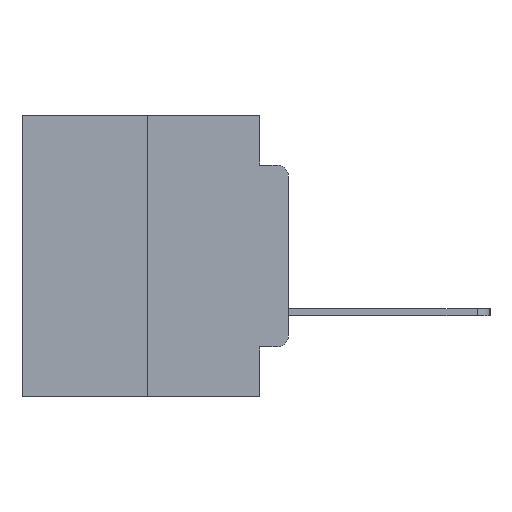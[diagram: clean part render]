
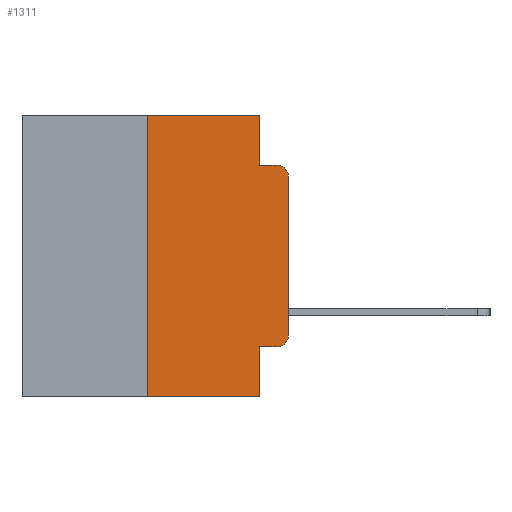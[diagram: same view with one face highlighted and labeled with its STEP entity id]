
A CAD part, left-side view. The second image highlights one B-rep face of the part: STEP entity #1311.
In plain terms, the highlighted planar face has unit normal (-1, 0, 0).
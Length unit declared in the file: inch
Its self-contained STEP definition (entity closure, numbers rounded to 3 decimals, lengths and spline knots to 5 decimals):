
#98 = DIRECTION ( 'NONE',  ( 1., 0., 0. ) ) ;
#114 = DIRECTION ( 'NONE',  ( 0., -1., 0. ) ) ;
#141 = ORIENTED_EDGE ( 'NONE', *, *, #3497, .T. ) ;
#243 = CIRCLE ( 'NONE', #25895, 0.02 ) ;
#265 = ORIENTED_EDGE ( 'NONE', *, *, #6377, .T. ) ;
#320 = ORIENTED_EDGE ( 'NONE', *, *, #17636, .F. ) ;
#381 = FACE_OUTER_BOUND ( 'NONE', #6805, .T. ) ;
#661 = ORIENTED_EDGE ( 'NONE', *, *, #2000, .F. ) ;
#1247 = PLANE ( 'NONE',  #13559 ) ;
#1311 = ADVANCED_FACE ( 'NONE', ( #381 ), #1247, .F. ) ;
#2000 = EDGE_CURVE ( 'NONE', #14058, #24439, #23608, .T. ) ;
#2503 = LINE ( 'NONE', #15978, #13134 ) ;
#2613 = CARTESIAN_POINT ( 'NONE',  ( 0., 0.02, -0.1085 ) ) ;
#2780 = ORIENTED_EDGE ( 'NONE', *, *, #16126, .F. ) ;
#3058 = DIRECTION ( 'NONE',  ( 0., 0., -1. ) ) ;
#3257 = LINE ( 'NONE', #22811, #13185 ) ;
#3497 = EDGE_CURVE ( 'NONE', #26567, #24439, #243, .T. ) ;
#3985 = ORIENTED_EDGE ( 'NONE', *, *, #16803, .T. ) ;
#5022 = ORIENTED_EDGE ( 'NONE', *, *, #11822, .T. ) ;
#5817 = CARTESIAN_POINT ( 'NONE',  ( 0., 0., 0. ) ) ;
#5820 = CIRCLE ( 'NONE', #22094, 0.02 ) ;
#6288 = ORIENTED_EDGE ( 'NONE', *, *, #12007, .F. ) ;
#6369 = VERTEX_POINT ( 'NONE', #16128 ) ;
#6377 = EDGE_CURVE ( 'NONE', #10639, #26567, #12875, .T. ) ;
#6389 = DIRECTION ( 'NONE',  ( -1., 0., 0. ) ) ;
#6685 = CARTESIAN_POINT ( 'NONE',  ( 0., 0.051, -0.0885 ) ) ;
#6805 = EDGE_LOOP ( 'NONE', ( #265, #141, #661, #320, #2780, #17158, #8046, #6288, #5022, #3985 ) ) ;
#8046 = ORIENTED_EDGE ( 'NONE', *, *, #18594, .T. ) ;
#8065 = LINE ( 'NONE', #21687, #18872 ) ;
#8279 = VECTOR ( 'NONE', #17229, 39.37008 ) ;
#8461 = VERTEX_POINT ( 'NONE', #20288 ) ;
#9256 = VECTOR ( 'NONE', #12437, 39.37008 ) ;
#9667 = DIRECTION ( 'NONE',  ( 0., 0., 1. ) ) ;
#10191 = CARTESIAN_POINT ( 'NONE',  ( 0., 0.473, 0. ) ) ;
#10449 = EDGE_CURVE ( 'NONE', #10843, #10741, #8065, .T. ) ;
#10500 = VECTOR ( 'NONE', #26169, 39.37008 ) ;
#10639 = VERTEX_POINT ( 'NONE', #12827 ) ;
#10712 = CARTESIAN_POINT ( 'NONE',  ( 0., 0.02, -0.0885 ) ) ;
#10741 = VERTEX_POINT ( 'NONE', #15293 ) ;
#10785 = CARTESIAN_POINT ( 'NONE',  ( 0., 0.02, -0.3915 ) ) ;
#10843 = VERTEX_POINT ( 'NONE', #21673 ) ;
#10846 = DIRECTION ( 'NONE',  ( 0., 0., -1. ) ) ;
#10914 = VERTEX_POINT ( 'NONE', #23831 ) ;
#11822 = EDGE_CURVE ( 'NONE', #6369, #10914, #25566, .T. ) ;
#12007 = EDGE_CURVE ( 'NONE', #6369, #8461, #19999, .T. ) ;
#12437 = DIRECTION ( 'NONE',  ( 0., 0., -1. ) ) ;
#12827 = CARTESIAN_POINT ( 'NONE',  ( 0., 0., -0.3915 ) ) ;
#12865 = DIRECTION ( 'NONE',  ( 0., 0., -1. ) ) ;
#12875 = LINE ( 'NONE', #5817, #18181 ) ;
#13042 = VECTOR ( 'NONE', #114, 39.37008 ) ;
#13134 = VECTOR ( 'NONE', #15884, 39.37008 ) ;
#13185 = VECTOR ( 'NONE', #10846, 39.37008 ) ;
#13559 = AXIS2_PLACEMENT_3D ( 'NONE', #16146, #98, #3058 ) ;
#13990 = VERTEX_POINT ( 'NONE', #14558 ) ;
#14058 = VERTEX_POINT ( 'NONE', #16714 ) ;
#14147 = DIRECTION ( 'NONE',  ( 0., 0., 1. ) ) ;
#14558 = CARTESIAN_POINT ( 'NONE',  ( 0., 0.051, 0. ) ) ;
#15293 = CARTESIAN_POINT ( 'NONE',  ( 0., 0.25, 0. ) ) ;
#15331 = CARTESIAN_POINT ( 'NONE',  ( 0., 0.051, -0.4115 ) ) ;
#15884 = DIRECTION ( 'NONE',  ( 0., -1., 0. ) ) ;
#15978 = CARTESIAN_POINT ( 'NONE',  ( 0., 0.473, -0.5 ) ) ;
#16126 = EDGE_CURVE ( 'NONE', #10741, #13990, #26400, .T. ) ;
#16128 = CARTESIAN_POINT ( 'NONE',  ( 0., 0.051, -0.4115 ) ) ;
#16146 = CARTESIAN_POINT ( 'NONE',  ( 0., 0.473, 0. ) ) ;
#16714 = CARTESIAN_POINT ( 'NONE',  ( 0., 0.051, -0.0885 ) ) ;
#16803 = EDGE_CURVE ( 'NONE', #10914, #10639, #5820, .T. ) ;
#17158 = ORIENTED_EDGE ( 'NONE', *, *, #10449, .F. ) ;
#17229 = DIRECTION ( 'NONE',  ( 0., -1., 0. ) ) ;
#17636 = EDGE_CURVE ( 'NONE', #13990, #14058, #3257, .T. ) ;
#18181 = VECTOR ( 'NONE', #14147, 39.37008 ) ;
#18594 = EDGE_CURVE ( 'NONE', #10843, #8461, #2503, .T. ) ;
#18872 = VECTOR ( 'NONE', #9667, 39.37008 ) ;
#19999 = LINE ( 'NONE', #24340, #9256 ) ;
#20288 = CARTESIAN_POINT ( 'NONE',  ( 0., 0.051, -0.5 ) ) ;
#20666 = DIRECTION ( 'NONE',  ( 0., 0., -1. ) ) ;
#21133 = CARTESIAN_POINT ( 'NONE',  ( 0., 0., -0.1085 ) ) ;
#21673 = CARTESIAN_POINT ( 'NONE',  ( 0., 0.25, -0.5 ) ) ;
#21687 = CARTESIAN_POINT ( 'NONE',  ( 0., 0.25, 0. ) ) ;
#22094 = AXIS2_PLACEMENT_3D ( 'NONE', #10785, #24742, #12865 ) ;
#22811 = CARTESIAN_POINT ( 'NONE',  ( 0., 0.051, 0. ) ) ;
#23608 = LINE ( 'NONE', #6685, #13042 ) ;
#23831 = CARTESIAN_POINT ( 'NONE',  ( 0., 0.02, -0.4115 ) ) ;
#24340 = CARTESIAN_POINT ( 'NONE',  ( 0., 0.051, 0. ) ) ;
#24439 = VERTEX_POINT ( 'NONE', #10712 ) ;
#24742 = DIRECTION ( 'NONE',  ( -1., 0., 0. ) ) ;
#25566 = LINE ( 'NONE', #15331, #8279 ) ;
#25895 = AXIS2_PLACEMENT_3D ( 'NONE', #2613, #6389, #20666 ) ;
#26169 = DIRECTION ( 'NONE',  ( 0., -1., 0. ) ) ;
#26400 = LINE ( 'NONE', #10191, #10500 ) ;
#26567 = VERTEX_POINT ( 'NONE', #21133 ) ;
